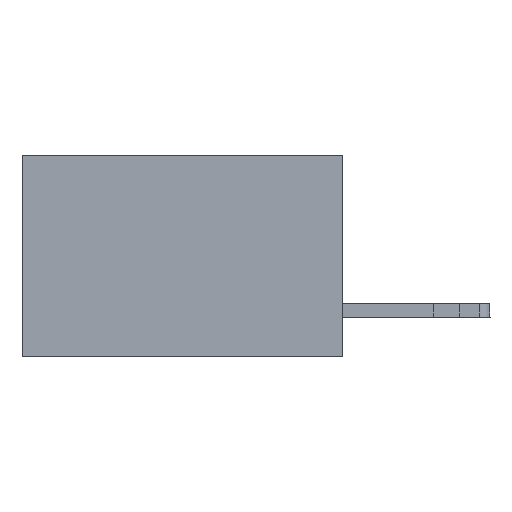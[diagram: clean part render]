
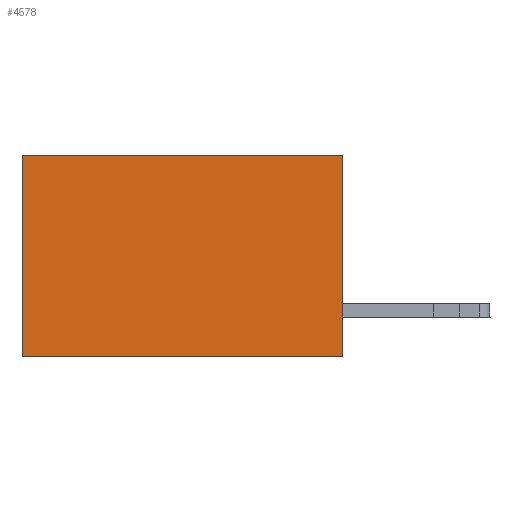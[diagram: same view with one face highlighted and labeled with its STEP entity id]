
A CAD part, left-side view. The second image highlights one B-rep face of the part: STEP entity #4578.
In plain terms, the highlighted planar face has unit normal (-1, 0, 0).
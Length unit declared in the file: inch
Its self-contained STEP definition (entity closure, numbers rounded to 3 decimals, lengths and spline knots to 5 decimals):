
#449 = CARTESIAN_POINT ( 'NONE',  ( 0.277, 0., -0.37 ) ) ;
#1060 = VECTOR ( 'NONE', #15799, 39.37008 ) ;
#1468 = CARTESIAN_POINT ( 'NONE',  ( 0.277, 0., 0. ) ) ;
#3183 = DIRECTION ( 'NONE',  ( 0., 1., 0. ) ) ;
#3523 = ORIENTED_EDGE ( 'NONE', *, *, #11557, .T. ) ;
#4576 = EDGE_CURVE ( 'NONE', #8538, #18451, #5696, .T. ) ;
#4578 = ADVANCED_FACE ( 'NONE', ( #7560 ), #13974, .F. ) ;
#4651 = VERTEX_POINT ( 'NONE', #17948 ) ;
#5696 = LINE ( 'NONE', #10663, #17217 ) ;
#5949 = EDGE_LOOP ( 'NONE', ( #3523, #21589, #6276, #13855 ) ) ;
#6276 = ORIENTED_EDGE ( 'NONE', *, *, #4576, .F. ) ;
#7560 = FACE_OUTER_BOUND ( 'NONE', #5949, .T. ) ;
#8538 = VERTEX_POINT ( 'NONE', #1468 ) ;
#9461 = AXIS2_PLACEMENT_3D ( 'NONE', #20716, #14287, #18953 ) ;
#9889 = VECTOR ( 'NONE', #3183, 39.37008 ) ;
#10550 = VERTEX_POINT ( 'NONE', #12348 ) ;
#10663 = CARTESIAN_POINT ( 'NONE',  ( 0.277, 0., -0.37 ) ) ;
#10727 = LINE ( 'NONE', #17460, #1060 ) ;
#11248 = EDGE_CURVE ( 'NONE', #18451, #4651, #10727, .T. ) ;
#11557 = EDGE_CURVE ( 'NONE', #10550, #4651, #20855, .T. ) ;
#11884 = EDGE_CURVE ( 'NONE', #8538, #10550, #21744, .T. ) ;
#12348 = CARTESIAN_POINT ( 'NONE',  ( 0.277, 0.59, 0. ) ) ;
#13855 = ORIENTED_EDGE ( 'NONE', *, *, #11884, .T. ) ;
#13974 = PLANE ( 'NONE',  #9461 ) ;
#14287 = DIRECTION ( 'NONE',  ( 1., 0., 0. ) ) ;
#15772 = CARTESIAN_POINT ( 'NONE',  ( 0.277, 0.59, -0.37 ) ) ;
#15799 = DIRECTION ( 'NONE',  ( 0., 1., 0. ) ) ;
#16059 = DIRECTION ( 'NONE',  ( 0., 0., -1. ) ) ;
#16913 = VECTOR ( 'NONE', #18873, 39.37008 ) ;
#17217 = VECTOR ( 'NONE', #16059, 39.37008 ) ;
#17460 = CARTESIAN_POINT ( 'NONE',  ( 0.277, 0., -0.37 ) ) ;
#17948 = CARTESIAN_POINT ( 'NONE',  ( 0.277, 0.59, -0.37 ) ) ;
#18451 = VERTEX_POINT ( 'NONE', #449 ) ;
#18873 = DIRECTION ( 'NONE',  ( 0., 0., -1. ) ) ;
#18953 = DIRECTION ( 'NONE',  ( 0., 0., -1. ) ) ;
#20716 = CARTESIAN_POINT ( 'NONE',  ( 0.277, 0., -0.37 ) ) ;
#20855 = LINE ( 'NONE', #15772, #16913 ) ;
#21526 = CARTESIAN_POINT ( 'NONE',  ( 0.277, 0., 0. ) ) ;
#21589 = ORIENTED_EDGE ( 'NONE', *, *, #11248, .F. ) ;
#21744 = LINE ( 'NONE', #21526, #9889 ) ;
